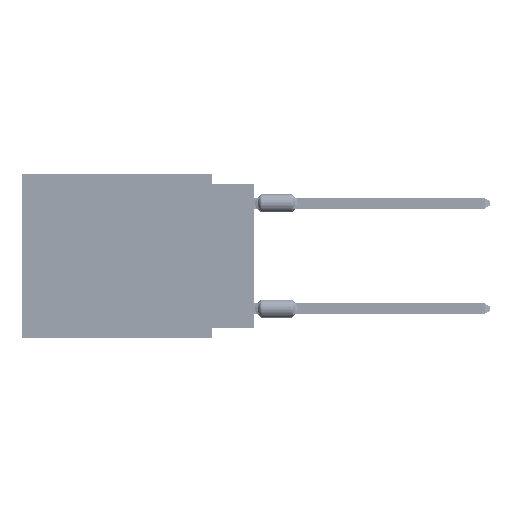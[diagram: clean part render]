
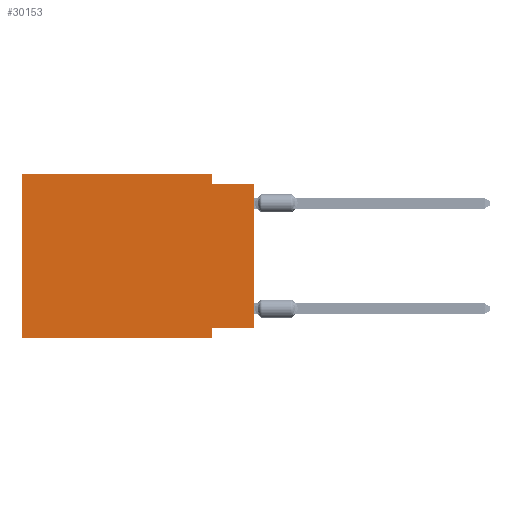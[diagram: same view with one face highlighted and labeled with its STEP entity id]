
A CAD part, left-side view. The second image highlights one B-rep face of the part: STEP entity #30153.
In plain terms, the highlighted planar face has unit normal (-1, 0, 0).
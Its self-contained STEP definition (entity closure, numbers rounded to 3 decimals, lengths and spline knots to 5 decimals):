
#1132 = EDGE_LOOP ( 'NONE', ( #44821, #37855, #61054, #59410, #3270, #68930, #66679, #21717 ) ) ;
#1274 = DIRECTION ( 'NONE',  ( 0., -1., 0. ) ) ;
#2818 = DIRECTION ( 'NONE',  ( 0., 0., 1. ) ) ;
#3270 = ORIENTED_EDGE ( 'NONE', *, *, #34637, .F. ) ;
#3909 = CARTESIAN_POINT ( 'NONE',  ( 0., 0.55, -0.39 ) ) ;
#4259 = EDGE_CURVE ( 'NONE', #56364, #44324, #36927, .T. ) ;
#6669 = VECTOR ( 'NONE', #39589, 39.37008 ) ;
#7109 = EDGE_CURVE ( 'NONE', #47117, #10891, #37405, .T. ) ;
#8975 = CARTESIAN_POINT ( 'NONE',  ( 0., 0.55, 0. ) ) ;
#9398 = VECTOR ( 'NONE', #2818, 39.37008 ) ;
#9528 = DIRECTION ( 'NONE',  ( 0., 0., -1. ) ) ;
#10891 = VERTEX_POINT ( 'NONE', #43474 ) ;
#10962 = VECTOR ( 'NONE', #34130, 39.37008 ) ;
#11525 = VECTOR ( 'NONE', #9528, 39.37008 ) ;
#11667 = LINE ( 'NONE', #35020, #18107 ) ;
#13799 = FACE_OUTER_BOUND ( 'NONE', #1132, .T. ) ;
#16415 = CARTESIAN_POINT ( 'NONE',  ( 0., 0.55, 0. ) ) ;
#17050 = CARTESIAN_POINT ( 'NONE',  ( 0., 0.55, 0. ) ) ;
#18107 = VECTOR ( 'NONE', #1274, 39.37008 ) ;
#19848 = DIRECTION ( 'NONE',  ( 0., 1., 0. ) ) ;
#20203 = CARTESIAN_POINT ( 'NONE',  ( 0., 0., -0.365 ) ) ;
#20443 = DIRECTION ( 'NONE',  ( 0., 0., -1. ) ) ;
#21213 = EDGE_CURVE ( 'NONE', #56364, #47117, #25400, .T. ) ;
#21717 = ORIENTED_EDGE ( 'NONE', *, *, #21213, .F. ) ;
#22965 = CARTESIAN_POINT ( 'NONE',  ( 0., 0.55, -0.39 ) ) ;
#23461 = EDGE_CURVE ( 'NONE', #47455, #10891, #28912, .T. ) ;
#25400 = LINE ( 'NONE', #20203, #66041 ) ;
#28539 = DIRECTION ( 'NONE',  ( 0., -1., 0. ) ) ;
#28912 = LINE ( 'NONE', #22965, #49652 ) ;
#30153 = ADVANCED_FACE ( 'NONE', ( #13799 ), #47543, .F. ) ;
#32853 = AXIS2_PLACEMENT_3D ( 'NONE', #8975, #53109, #20443 ) ;
#33289 = CARTESIAN_POINT ( 'NONE',  ( 0., 0., -0.025 ) ) ;
#33655 = LINE ( 'NONE', #39215, #6669 ) ;
#34130 = DIRECTION ( 'NONE',  ( 0., 0., 1. ) ) ;
#34218 = VERTEX_POINT ( 'NONE', #16415 ) ;
#34637 = EDGE_CURVE ( 'NONE', #47455, #34218, #67825, .T. ) ;
#34969 = CARTESIAN_POINT ( 'NONE',  ( 0., 0.1, 0. ) ) ;
#35020 = CARTESIAN_POINT ( 'NONE',  ( 0., 0.55, 0. ) ) ;
#35030 = CARTESIAN_POINT ( 'NONE',  ( 0., 0.1, -0.025 ) ) ;
#36189 = CARTESIAN_POINT ( 'NONE',  ( 0., 0., 0. ) ) ;
#36927 = LINE ( 'NONE', #36189, #9398 ) ;
#37405 = LINE ( 'NONE', #48878, #47347 ) ;
#37855 = ORIENTED_EDGE ( 'NONE', *, *, #54861, .F. ) ;
#39215 = CARTESIAN_POINT ( 'NONE',  ( 0., 0., -0.025 ) ) ;
#39589 = DIRECTION ( 'NONE',  ( 0., -1., 0. ) ) ;
#42598 = CARTESIAN_POINT ( 'NONE',  ( 0., 0., -0.365 ) ) ;
#43474 = CARTESIAN_POINT ( 'NONE',  ( 0., 0.1, -0.39 ) ) ;
#44324 = VERTEX_POINT ( 'NONE', #33289 ) ;
#44418 = DIRECTION ( 'NONE',  ( 0., 0., -1. ) ) ;
#44821 = ORIENTED_EDGE ( 'NONE', *, *, #4259, .T. ) ;
#47117 = VERTEX_POINT ( 'NONE', #66982 ) ;
#47347 = VECTOR ( 'NONE', #44418, 39.37008 ) ;
#47455 = VERTEX_POINT ( 'NONE', #3909 ) ;
#47543 = PLANE ( 'NONE',  #32853 ) ;
#48878 = CARTESIAN_POINT ( 'NONE',  ( 0., 0.1, -0.39 ) ) ;
#49652 = VECTOR ( 'NONE', #28539, 39.37008 ) ;
#50892 = EDGE_CURVE ( 'NONE', #34218, #61023, #11667, .T. ) ;
#53109 = DIRECTION ( 'NONE',  ( 1., 0., 0. ) ) ;
#54861 = EDGE_CURVE ( 'NONE', #55456, #44324, #33655, .T. ) ;
#55456 = VERTEX_POINT ( 'NONE', #35030 ) ;
#55484 = LINE ( 'NONE', #71762, #11525 ) ;
#56364 = VERTEX_POINT ( 'NONE', #42598 ) ;
#58707 = EDGE_CURVE ( 'NONE', #61023, #55456, #55484, .T. ) ;
#59410 = ORIENTED_EDGE ( 'NONE', *, *, #50892, .F. ) ;
#61023 = VERTEX_POINT ( 'NONE', #34969 ) ;
#61054 = ORIENTED_EDGE ( 'NONE', *, *, #58707, .F. ) ;
#66041 = VECTOR ( 'NONE', #19848, 39.37008 ) ;
#66679 = ORIENTED_EDGE ( 'NONE', *, *, #7109, .F. ) ;
#66982 = CARTESIAN_POINT ( 'NONE',  ( 0., 0.1, -0.365 ) ) ;
#67825 = LINE ( 'NONE', #17050, #10962 ) ;
#68930 = ORIENTED_EDGE ( 'NONE', *, *, #23461, .T. ) ;
#71762 = CARTESIAN_POINT ( 'NONE',  ( 0., 0.1, 0. ) ) ;
